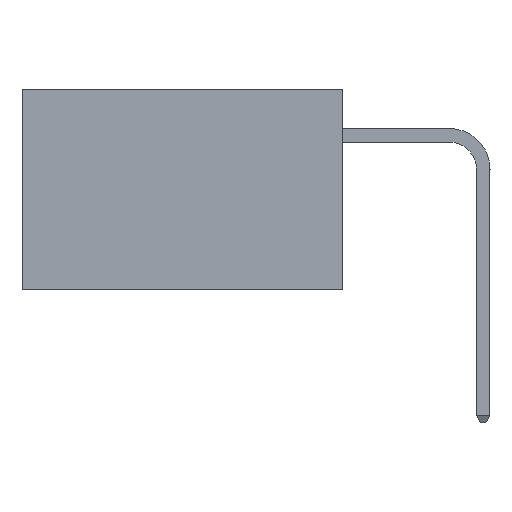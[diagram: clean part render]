
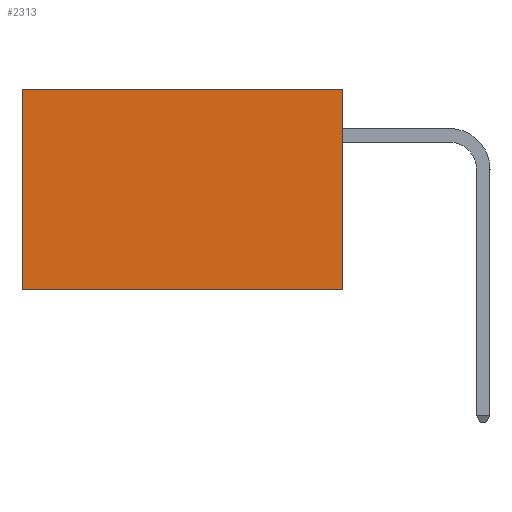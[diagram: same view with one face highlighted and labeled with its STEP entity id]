
A CAD part, left-side view. The second image highlights one B-rep face of the part: STEP entity #2313.
In plain terms, the highlighted planar face has unit normal (-1, 0, 0).
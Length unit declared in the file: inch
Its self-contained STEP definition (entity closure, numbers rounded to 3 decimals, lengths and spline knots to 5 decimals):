
#1244 = CARTESIAN_POINT ( 'NONE',  ( 0.277, 0., -0.37 ) ) ;
#1823 = CARTESIAN_POINT ( 'NONE',  ( 0.277, 0., 0. ) ) ;
#2313 = ADVANCED_FACE ( 'NONE', ( #5279 ), #8106, .F. ) ;
#3507 = CARTESIAN_POINT ( 'NONE',  ( 0.277, 0.59, -0.37 ) ) ;
#3540 = VECTOR ( 'NONE', #23661, 39.37008 ) ;
#3702 = DIRECTION ( 'NONE',  ( 0., 0., -1. ) ) ;
#4807 = VECTOR ( 'NONE', #15465, 39.37008 ) ;
#5279 = FACE_OUTER_BOUND ( 'NONE', #18449, .T. ) ;
#5376 = ORIENTED_EDGE ( 'NONE', *, *, #5383, .T. ) ;
#5383 = EDGE_CURVE ( 'NONE', #7802, #12767, #10569, .T. ) ;
#6950 = VERTEX_POINT ( 'NONE', #20398 ) ;
#7802 = VERTEX_POINT ( 'NONE', #7958 ) ;
#7958 = CARTESIAN_POINT ( 'NONE',  ( 0.277, 0.59, 0. ) ) ;
#8106 = PLANE ( 'NONE',  #9720 ) ;
#8665 = EDGE_CURVE ( 'NONE', #6950, #12767, #10046, .T. ) ;
#9720 = AXIS2_PLACEMENT_3D ( 'NONE', #1244, #22660, #3702 ) ;
#9721 = VECTOR ( 'NONE', #16986, 39.37008 ) ;
#10046 = LINE ( 'NONE', #14954, #3540 ) ;
#10364 = EDGE_CURVE ( 'NONE', #20337, #7802, #27070, .T. ) ;
#10569 = LINE ( 'NONE', #13299, #4807 ) ;
#10980 = CARTESIAN_POINT ( 'NONE',  ( 0.277, 0., 0. ) ) ;
#12767 = VERTEX_POINT ( 'NONE', #3507 ) ;
#13240 = DIRECTION ( 'NONE',  ( 0., 0., -1. ) ) ;
#13299 = CARTESIAN_POINT ( 'NONE',  ( 0.277, 0.59, -0.37 ) ) ;
#14954 = CARTESIAN_POINT ( 'NONE',  ( 0.277, 0., -0.37 ) ) ;
#15465 = DIRECTION ( 'NONE',  ( 0., 0., -1. ) ) ;
#16986 = DIRECTION ( 'NONE',  ( 0., 1., 0. ) ) ;
#18449 = EDGE_LOOP ( 'NONE', ( #5376, #20558, #20763, #26412 ) ) ;
#20337 = VERTEX_POINT ( 'NONE', #10980 ) ;
#20366 = LINE ( 'NONE', #24112, #24793 ) ;
#20398 = CARTESIAN_POINT ( 'NONE',  ( 0.277, 0., -0.37 ) ) ;
#20558 = ORIENTED_EDGE ( 'NONE', *, *, #8665, .F. ) ;
#20763 = ORIENTED_EDGE ( 'NONE', *, *, #26042, .F. ) ;
#22660 = DIRECTION ( 'NONE',  ( 1., 0., 0. ) ) ;
#23661 = DIRECTION ( 'NONE',  ( 0., 1., 0. ) ) ;
#24112 = CARTESIAN_POINT ( 'NONE',  ( 0.277, 0., -0.37 ) ) ;
#24793 = VECTOR ( 'NONE', #13240, 39.37008 ) ;
#26042 = EDGE_CURVE ( 'NONE', #20337, #6950, #20366, .T. ) ;
#26412 = ORIENTED_EDGE ( 'NONE', *, *, #10364, .T. ) ;
#27070 = LINE ( 'NONE', #1823, #9721 ) ;
